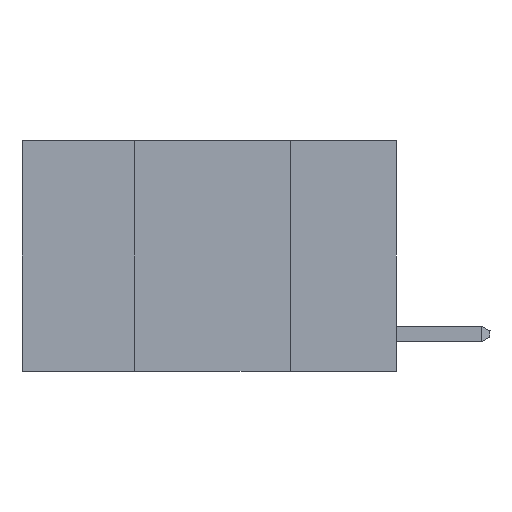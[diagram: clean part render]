
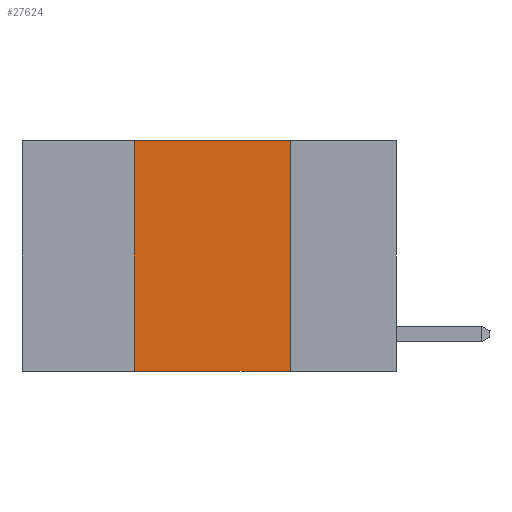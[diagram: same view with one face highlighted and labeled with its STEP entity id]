
A CAD part, left-side view. The second image highlights one B-rep face of the part: STEP entity #27624.
In plain terms, the highlighted planar face has unit normal (-1, 0, 0).
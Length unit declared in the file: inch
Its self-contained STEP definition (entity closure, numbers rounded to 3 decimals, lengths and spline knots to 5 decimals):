
#433 = EDGE_LOOP ( 'NONE', ( #4699, #16200, #22253, #26847 ) ) ;
#1993 = DIRECTION ( 'NONE',  ( 0., -1., 0. ) ) ;
#2065 = CARTESIAN_POINT ( 'NONE',  ( 0., 0.17, -0.37 ) ) ;
#2563 = VECTOR ( 'NONE', #25103, 39.37008 ) ;
#3009 = CARTESIAN_POINT ( 'NONE',  ( 0., 0.17, 0. ) ) ;
#3809 = EDGE_CURVE ( 'NONE', #14290, #7086, #4188, .T. ) ;
#4188 = LINE ( 'NONE', #4481, #19437 ) ;
#4481 = CARTESIAN_POINT ( 'NONE',  ( 0., 0.6, 0. ) ) ;
#4635 = VERTEX_POINT ( 'NONE', #2065 ) ;
#4699 = ORIENTED_EDGE ( 'NONE', *, *, #6116, .F. ) ;
#4761 = CARTESIAN_POINT ( 'NONE',  ( 0., 0.6, -0.37 ) ) ;
#5413 = DIRECTION ( 'NONE',  ( 0., 0., -1. ) ) ;
#5689 = EDGE_CURVE ( 'NONE', #23363, #14290, #17762, .T. ) ;
#6116 = EDGE_CURVE ( 'NONE', #7086, #4635, #14541, .T. ) ;
#6191 = CARTESIAN_POINT ( 'NONE',  ( 0., 0.6, 0. ) ) ;
#7086 = VERTEX_POINT ( 'NONE', #3009 ) ;
#9654 = EDGE_CURVE ( 'NONE', #23363, #4635, #24966, .T. ) ;
#12484 = CARTESIAN_POINT ( 'NONE',  ( 0., 0.17, 0. ) ) ;
#14290 = VERTEX_POINT ( 'NONE', #26401 ) ;
#14541 = LINE ( 'NONE', #12484, #27420 ) ;
#15155 = VECTOR ( 'NONE', #24393, 39.37008 ) ;
#15405 = CARTESIAN_POINT ( 'NONE',  ( 0., 0.42, 0. ) ) ;
#16200 = ORIENTED_EDGE ( 'NONE', *, *, #3809, .F. ) ;
#17762 = LINE ( 'NONE', #15405, #15155 ) ;
#19437 = VECTOR ( 'NONE', #1993, 39.37008 ) ;
#21551 = DIRECTION ( 'NONE',  ( 1., 0., 0. ) ) ;
#22253 = ORIENTED_EDGE ( 'NONE', *, *, #5689, .F. ) ;
#23363 = VERTEX_POINT ( 'NONE', #25163 ) ;
#23617 = DIRECTION ( 'NONE',  ( 0., 0., -1. ) ) ;
#24048 = FACE_OUTER_BOUND ( 'NONE', #433, .T. ) ;
#24393 = DIRECTION ( 'NONE',  ( 0., 0., 1. ) ) ;
#24966 = LINE ( 'NONE', #4761, #2563 ) ;
#25103 = DIRECTION ( 'NONE',  ( 0., -1., 0. ) ) ;
#25163 = CARTESIAN_POINT ( 'NONE',  ( 0., 0.42, -0.37 ) ) ;
#26401 = CARTESIAN_POINT ( 'NONE',  ( 0., 0.42, 0. ) ) ;
#26410 = PLANE ( 'NONE',  #26582 ) ;
#26582 = AXIS2_PLACEMENT_3D ( 'NONE', #6191, #21551, #23617 ) ;
#26847 = ORIENTED_EDGE ( 'NONE', *, *, #9654, .T. ) ;
#27420 = VECTOR ( 'NONE', #5413, 39.37008 ) ;
#27624 = ADVANCED_FACE ( 'NONE', ( #24048 ), #26410, .F. ) ;
